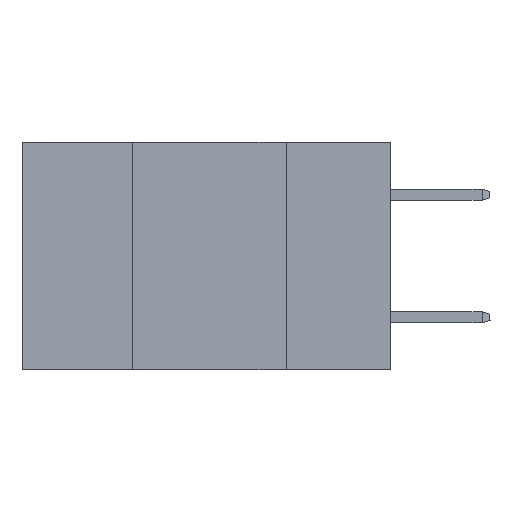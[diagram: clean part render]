
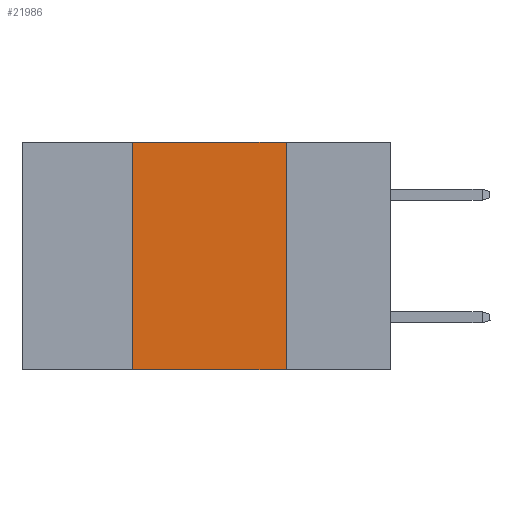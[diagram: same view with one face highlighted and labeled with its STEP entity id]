
A CAD part, left-side view. The second image highlights one B-rep face of the part: STEP entity #21986.
In plain terms, the highlighted planar face has unit normal (-1, 0, 0).
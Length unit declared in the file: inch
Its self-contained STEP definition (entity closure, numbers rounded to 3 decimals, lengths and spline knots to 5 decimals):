
#904 = PLANE ( 'NONE',  #23182 ) ;
#1016 = VECTOR ( 'NONE', #32756, 39.37008 ) ;
#3375 = ORIENTED_EDGE ( 'NONE', *, *, #11188, .F. ) ;
#6497 = LINE ( 'NONE', #22269, #12339 ) ;
#7046 = LINE ( 'NONE', #32774, #20570 ) ;
#7799 = VERTEX_POINT ( 'NONE', #11259 ) ;
#8252 = VERTEX_POINT ( 'NONE', #37318 ) ;
#8619 = DIRECTION ( 'NONE',  ( 0., -1., 0. ) ) ;
#9001 = ORIENTED_EDGE ( 'NONE', *, *, #24538, .T. ) ;
#9230 = EDGE_CURVE ( 'NONE', #26091, #36439, #20551, .T. ) ;
#11188 = EDGE_CURVE ( 'NONE', #8252, #26091, #19570, .T. ) ;
#11259 = CARTESIAN_POINT ( 'NONE',  ( 0., 0.17, -0.37 ) ) ;
#11479 = DIRECTION ( 'NONE',  ( 1., 0., 0. ) ) ;
#12339 = VECTOR ( 'NONE', #32002, 39.37008 ) ;
#14289 = DIRECTION ( 'NONE',  ( 0., 0., -1. ) ) ;
#19570 = LINE ( 'NONE', #20203, #1016 ) ;
#20203 = CARTESIAN_POINT ( 'NONE',  ( 0., 0.42, 0. ) ) ;
#20551 = LINE ( 'NONE', #41904, #28451 ) ;
#20570 = VECTOR ( 'NONE', #36666, 39.37008 ) ;
#21986 = ADVANCED_FACE ( 'NONE', ( #28115 ), #904, .F. ) ;
#22269 = CARTESIAN_POINT ( 'NONE',  ( 0., 0.17, 0. ) ) ;
#23182 = AXIS2_PLACEMENT_3D ( 'NONE', #27908, #11479, #14289 ) ;
#24538 = EDGE_CURVE ( 'NONE', #8252, #7799, #7046, .T. ) ;
#25088 = CARTESIAN_POINT ( 'NONE',  ( 0., 0.17, 0. ) ) ;
#26091 = VERTEX_POINT ( 'NONE', #40979 ) ;
#27908 = CARTESIAN_POINT ( 'NONE',  ( 0., 0.6, 0. ) ) ;
#28115 = FACE_OUTER_BOUND ( 'NONE', #30869, .T. ) ;
#28451 = VECTOR ( 'NONE', #8619, 39.37008 ) ;
#30869 = EDGE_LOOP ( 'NONE', ( #41369, #38591, #3375, #9001 ) ) ;
#32002 = DIRECTION ( 'NONE',  ( 0., 0., -1. ) ) ;
#32756 = DIRECTION ( 'NONE',  ( 0., 0., 1. ) ) ;
#32774 = CARTESIAN_POINT ( 'NONE',  ( 0., 0.6, -0.37 ) ) ;
#36439 = VERTEX_POINT ( 'NONE', #25088 ) ;
#36561 = EDGE_CURVE ( 'NONE', #36439, #7799, #6497, .T. ) ;
#36666 = DIRECTION ( 'NONE',  ( 0., -1., 0. ) ) ;
#37318 = CARTESIAN_POINT ( 'NONE',  ( 0., 0.42, -0.37 ) ) ;
#38591 = ORIENTED_EDGE ( 'NONE', *, *, #9230, .F. ) ;
#40979 = CARTESIAN_POINT ( 'NONE',  ( 0., 0.42, 0. ) ) ;
#41369 = ORIENTED_EDGE ( 'NONE', *, *, #36561, .F. ) ;
#41904 = CARTESIAN_POINT ( 'NONE',  ( 0., 0.6, 0. ) ) ;
